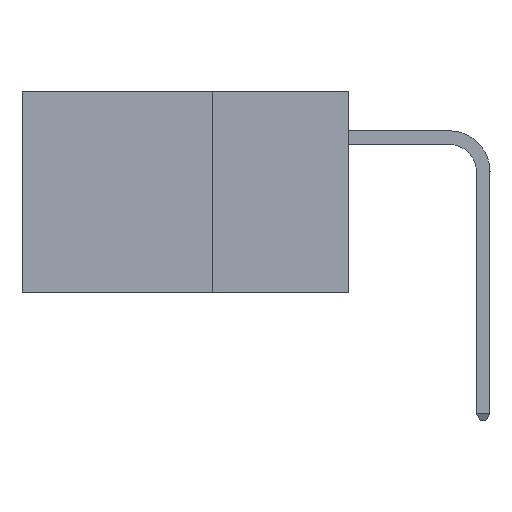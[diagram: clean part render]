
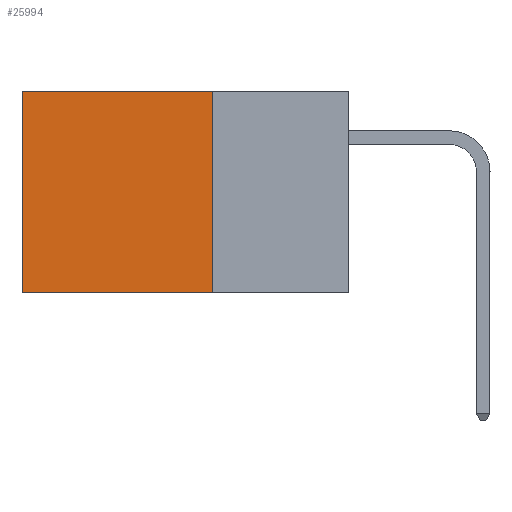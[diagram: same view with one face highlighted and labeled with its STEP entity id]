
A CAD part, left-side view. The second image highlights one B-rep face of the part: STEP entity #25994.
In plain terms, the highlighted planar face has unit normal (-1, 0, 0).
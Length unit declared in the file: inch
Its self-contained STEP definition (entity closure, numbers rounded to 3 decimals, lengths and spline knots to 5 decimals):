
#3019 = PLANE ( 'NONE',  #16589 ) ;
#3607 = CARTESIAN_POINT ( 'NONE',  ( 0.2875, 0.25, 0. ) ) ;
#4066 = CARTESIAN_POINT ( 'NONE',  ( 0.2875, 0.25, -0.37 ) ) ;
#4281 = VERTEX_POINT ( 'NONE', #34054 ) ;
#4796 = LINE ( 'NONE', #28730, #32620 ) ;
#5652 = CARTESIAN_POINT ( 'NONE',  ( 0.2875, 0.25, 0. ) ) ;
#5743 = EDGE_CURVE ( 'NONE', #25601, #4281, #19254, .T. ) ;
#6570 = EDGE_LOOP ( 'NONE', ( #29807, #28972, #30268, #9663 ) ) ;
#8534 = DIRECTION ( 'NONE',  ( 0., 1., 0. ) ) ;
#8777 = DIRECTION ( 'NONE',  ( 0., 0., -1. ) ) ;
#9232 = VECTOR ( 'NONE', #8534, 39.37008 ) ;
#9358 = DIRECTION ( 'NONE',  ( 0., 0., -1. ) ) ;
#9663 = ORIENTED_EDGE ( 'NONE', *, *, #28141, .T. ) ;
#13128 = VECTOR ( 'NONE', #20209, 39.37008 ) ;
#14120 = EDGE_CURVE ( 'NONE', #24343, #4281, #4796, .T. ) ;
#14677 = FACE_OUTER_BOUND ( 'NONE', #6570, .T. ) ;
#14726 = CARTESIAN_POINT ( 'NONE',  ( 0.2875, 0.25, 0. ) ) ;
#15323 = CARTESIAN_POINT ( 'NONE',  ( 0.2875, 0.6, 0. ) ) ;
#16096 = CARTESIAN_POINT ( 'NONE',  ( 0.2875, 0.25, -0.37 ) ) ;
#16176 = EDGE_CURVE ( 'NONE', #18686, #25601, #34249, .T. ) ;
#16589 = AXIS2_PLACEMENT_3D ( 'NONE', #22648, #25408, #8777 ) ;
#18686 = VERTEX_POINT ( 'NONE', #3607 ) ;
#19254 = LINE ( 'NONE', #16096, #33815 ) ;
#20209 = DIRECTION ( 'NONE',  ( 0., 0., -1. ) ) ;
#22648 = CARTESIAN_POINT ( 'NONE',  ( 0.2875, 0.25, 0. ) ) ;
#24343 = VERTEX_POINT ( 'NONE', #15323 ) ;
#25408 = DIRECTION ( 'NONE',  ( 1., 0., 0. ) ) ;
#25601 = VERTEX_POINT ( 'NONE', #4066 ) ;
#25994 = ADVANCED_FACE ( 'NONE', ( #14677 ), #3019, .F. ) ;
#28141 = EDGE_CURVE ( 'NONE', #18686, #24343, #31329, .T. ) ;
#28730 = CARTESIAN_POINT ( 'NONE',  ( 0.2875, 0.6, 0. ) ) ;
#28972 = ORIENTED_EDGE ( 'NONE', *, *, #5743, .F. ) ;
#29807 = ORIENTED_EDGE ( 'NONE', *, *, #14120, .T. ) ;
#30268 = ORIENTED_EDGE ( 'NONE', *, *, #16176, .F. ) ;
#31329 = LINE ( 'NONE', #5652, #9232 ) ;
#32620 = VECTOR ( 'NONE', #9358, 39.37008 ) ;
#33815 = VECTOR ( 'NONE', #35280, 39.37008 ) ;
#34054 = CARTESIAN_POINT ( 'NONE',  ( 0.2875, 0.6, -0.37 ) ) ;
#34249 = LINE ( 'NONE', #14726, #13128 ) ;
#35280 = DIRECTION ( 'NONE',  ( 0., 1., 0. ) ) ;
